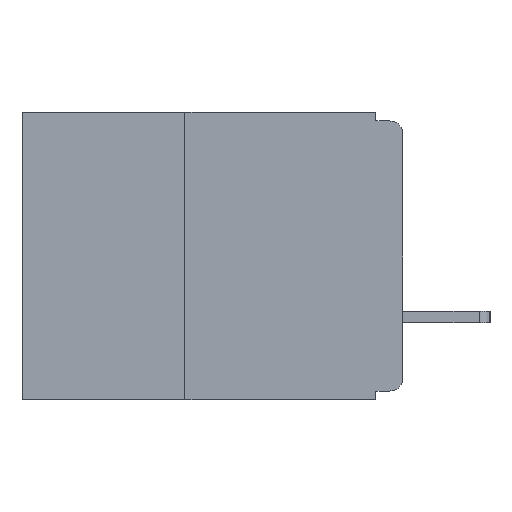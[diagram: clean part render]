
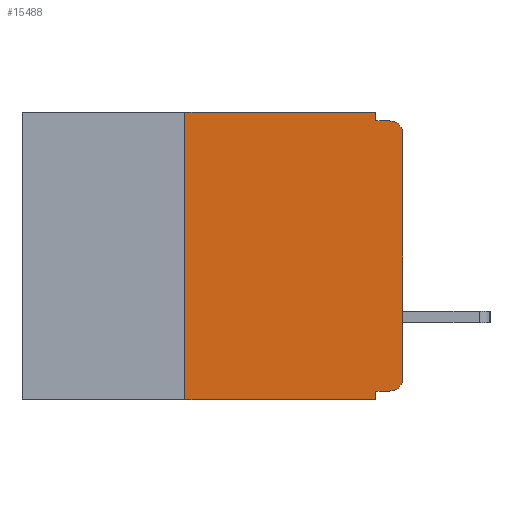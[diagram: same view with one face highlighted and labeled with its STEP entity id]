
A CAD part, left-side view. The second image highlights one B-rep face of the part: STEP entity #15488.
In plain terms, the highlighted planar face has unit normal (-1, 0, 0).
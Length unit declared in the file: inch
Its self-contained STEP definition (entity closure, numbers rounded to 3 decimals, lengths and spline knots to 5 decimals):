
#4 = EDGE_CURVE ( 'NONE', #972, #12404, #18686, .T. ) ;
#41 = CARTESIAN_POINT ( 'NONE',  ( 0., 0.031, 0. ) ) ;
#57 = DIRECTION ( 'NONE',  ( 0., -1., 0. ) ) ;
#244 = DIRECTION ( 'NONE',  ( 0., 0., -1. ) ) ;
#499 = EDGE_LOOP ( 'NONE', ( #10884, #3734, #1292, #8029, #1407, #15140, #16352, #3075, #610, #12489 ) ) ;
#610 = ORIENTED_EDGE ( 'NONE', *, *, #13265, .F. ) ;
#886 = LINE ( 'NONE', #19534, #12906 ) ;
#893 = EDGE_CURVE ( 'NONE', #972, #2778, #18319, .T. ) ;
#972 = VERTEX_POINT ( 'NONE', #19267 ) ;
#1292 = ORIENTED_EDGE ( 'NONE', *, *, #5202, .F. ) ;
#1335 = DIRECTION ( 'NONE',  ( 0., 0., 1. ) ) ;
#1407 = ORIENTED_EDGE ( 'NONE', *, *, #19734, .F. ) ;
#1413 = DIRECTION ( 'NONE',  ( 0., 0., -1. ) ) ;
#1787 = PLANE ( 'NONE',  #10918 ) ;
#2778 = VERTEX_POINT ( 'NONE', #4732 ) ;
#2965 = LINE ( 'NONE', #12570, #19108 ) ;
#3075 = ORIENTED_EDGE ( 'NONE', *, *, #4365, .F. ) ;
#3103 = VECTOR ( 'NONE', #9025, 39.37008 ) ;
#3363 = DIRECTION ( 'NONE',  ( 0., 0., -1. ) ) ;
#3734 = ORIENTED_EDGE ( 'NONE', *, *, #14168, .T. ) ;
#3756 = CARTESIAN_POINT ( 'NONE',  ( 0., 0.015, -0.025 ) ) ;
#4365 = EDGE_CURVE ( 'NONE', #11624, #12404, #7181, .T. ) ;
#4635 = CARTESIAN_POINT ( 'NONE',  ( 0., 0., -0.32 ) ) ;
#4732 = CARTESIAN_POINT ( 'NONE',  ( 0., 0.25, 0. ) ) ;
#5141 = AXIS2_PLACEMENT_3D ( 'NONE', #3756, #14747, #5335 ) ;
#5202 = EDGE_CURVE ( 'NONE', #9836, #5586, #2965, .T. ) ;
#5263 = CARTESIAN_POINT ( 'NONE',  ( 0., 0.031, -0.33 ) ) ;
#5335 = DIRECTION ( 'NONE',  ( 0., 0., -1. ) ) ;
#5392 = LINE ( 'NONE', #41, #5917 ) ;
#5521 = EDGE_CURVE ( 'NONE', #15418, #9836, #5392, .T. ) ;
#5586 = VERTEX_POINT ( 'NONE', #19248 ) ;
#5917 = VECTOR ( 'NONE', #244, 39.37008 ) ;
#6207 = CARTESIAN_POINT ( 'NONE',  ( 0., 0.25, -0.33 ) ) ;
#6323 = CARTESIAN_POINT ( 'NONE',  ( 0., 0., -0.305 ) ) ;
#6699 = VECTOR ( 'NONE', #18557, 39.37008 ) ;
#7072 = CARTESIAN_POINT ( 'NONE',  ( 0., 0.015, -0.32 ) ) ;
#7181 = LINE ( 'NONE', #18645, #6699 ) ;
#7453 = LINE ( 'NONE', #4635, #11090 ) ;
#7714 = VERTEX_POINT ( 'NONE', #14179 ) ;
#8029 = ORIENTED_EDGE ( 'NONE', *, *, #5521, .F. ) ;
#8050 = CARTESIAN_POINT ( 'NONE',  ( 0., 0.031, -0.01 ) ) ;
#8977 = EDGE_CURVE ( 'NONE', #9125, #7714, #15133, .T. ) ;
#9025 = DIRECTION ( 'NONE',  ( 0., 0., 1. ) ) ;
#9125 = VERTEX_POINT ( 'NONE', #6323 ) ;
#9836 = VERTEX_POINT ( 'NONE', #8050 ) ;
#9974 = VECTOR ( 'NONE', #1335, 39.37008 ) ;
#10727 = VERTEX_POINT ( 'NONE', #7072 ) ;
#10775 = DIRECTION ( 'NONE',  ( -1., 0., 0. ) ) ;
#10884 = ORIENTED_EDGE ( 'NONE', *, *, #8977, .T. ) ;
#10918 = AXIS2_PLACEMENT_3D ( 'NONE', #18974, #12754, #3363 ) ;
#10995 = FACE_OUTER_BOUND ( 'NONE', #499, .T. ) ;
#11032 = CARTESIAN_POINT ( 'NONE',  ( 0., 0.031, 0. ) ) ;
#11090 = VECTOR ( 'NONE', #17190, 39.37008 ) ;
#11624 = VERTEX_POINT ( 'NONE', #12432 ) ;
#12404 = VERTEX_POINT ( 'NONE', #5263 ) ;
#12432 = CARTESIAN_POINT ( 'NONE',  ( 0., 0.031, -0.32 ) ) ;
#12489 = ORIENTED_EDGE ( 'NONE', *, *, #13227, .T. ) ;
#12491 = DIRECTION ( 'NONE',  ( 0., -1., 0. ) ) ;
#12570 = CARTESIAN_POINT ( 'NONE',  ( 0., 0., -0.01 ) ) ;
#12754 = DIRECTION ( 'NONE',  ( 1., 0., 0. ) ) ;
#12906 = VECTOR ( 'NONE', #18080, 39.37008 ) ;
#13227 = EDGE_CURVE ( 'NONE', #10727, #9125, #14561, .T. ) ;
#13265 = EDGE_CURVE ( 'NONE', #10727, #11624, #7453, .T. ) ;
#14043 = AXIS2_PLACEMENT_3D ( 'NONE', #20092, #10775, #1413 ) ;
#14168 = EDGE_CURVE ( 'NONE', #7714, #5586, #15752, .T. ) ;
#14179 = CARTESIAN_POINT ( 'NONE',  ( 0., 0., -0.025 ) ) ;
#14561 = CIRCLE ( 'NONE', #14043, 0.015 ) ;
#14747 = DIRECTION ( 'NONE',  ( -1., 0., 0. ) ) ;
#15133 = LINE ( 'NONE', #18413, #3103 ) ;
#15140 = ORIENTED_EDGE ( 'NONE', *, *, #893, .F. ) ;
#15418 = VERTEX_POINT ( 'NONE', #11032 ) ;
#15488 = ADVANCED_FACE ( 'NONE', ( #10995 ), #1787, .F. ) ;
#15752 = CIRCLE ( 'NONE', #5141, 0.015 ) ;
#16352 = ORIENTED_EDGE ( 'NONE', *, *, #4, .T. ) ;
#16391 = CARTESIAN_POINT ( 'NONE',  ( 0., 0.437, -0.33 ) ) ;
#17190 = DIRECTION ( 'NONE',  ( 0., 1., 0. ) ) ;
#18080 = DIRECTION ( 'NONE',  ( 0., -1., 0. ) ) ;
#18196 = VECTOR ( 'NONE', #57, 39.37008 ) ;
#18319 = LINE ( 'NONE', #6207, #9974 ) ;
#18413 = CARTESIAN_POINT ( 'NONE',  ( 0., 0., 0. ) ) ;
#18557 = DIRECTION ( 'NONE',  ( 0., 0., -1. ) ) ;
#18645 = CARTESIAN_POINT ( 'NONE',  ( 0., 0.031, -0.33 ) ) ;
#18686 = LINE ( 'NONE', #16391, #18196 ) ;
#18974 = CARTESIAN_POINT ( 'NONE',  ( 0., 0.437, 0. ) ) ;
#19108 = VECTOR ( 'NONE', #12491, 39.37008 ) ;
#19248 = CARTESIAN_POINT ( 'NONE',  ( 0., 0.015, -0.01 ) ) ;
#19267 = CARTESIAN_POINT ( 'NONE',  ( 0., 0.25, -0.33 ) ) ;
#19534 = CARTESIAN_POINT ( 'NONE',  ( 0., 0.437, 0. ) ) ;
#19734 = EDGE_CURVE ( 'NONE', #2778, #15418, #886, .T. ) ;
#20092 = CARTESIAN_POINT ( 'NONE',  ( 0., 0.015, -0.305 ) ) ;
